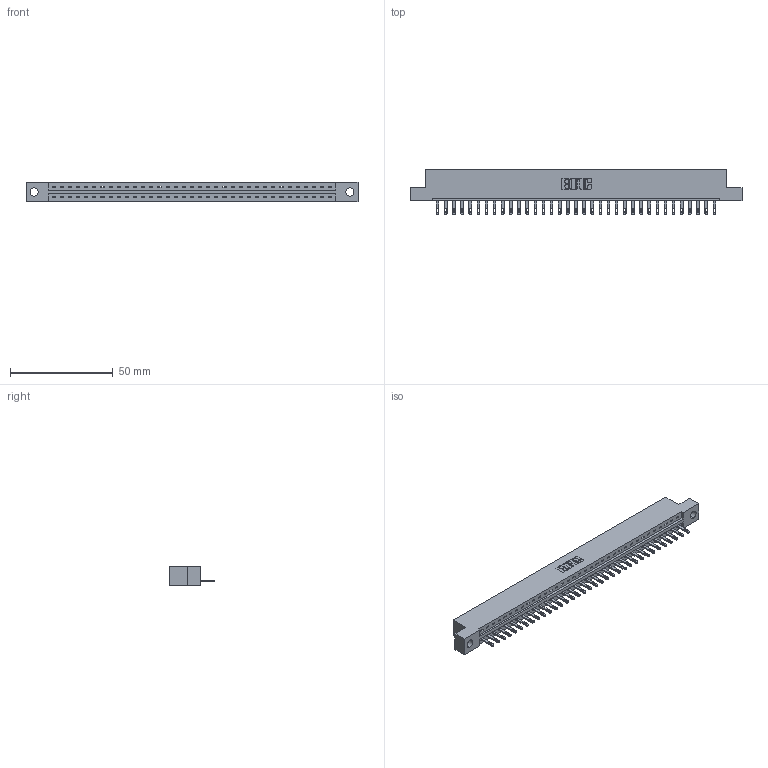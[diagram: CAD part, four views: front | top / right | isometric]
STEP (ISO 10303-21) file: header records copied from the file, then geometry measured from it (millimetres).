
FILE_DESCRIPTION (( 'STEP AP203' ), '1' );
FILE_NAME ('337-035-500-104.STEP', '2019-10-01T12:21:12', ( '' ), ( '' ), 'SwSTEP 2.0', 'SolidWorks 2016', '' );
FILE_SCHEMA (( 'CONFIG_CONTROL_DESIGN' ));
Length unit declared in the file: inch
Products named in the file (3): 337 Part_Flush Mounting Lugs - 0.156 Dia-TH; 337-035-500-104; 345-292-001_345-293-100
Assembly tree (36 placements, depth 2):
  337-035-500-104
    337 Part_Flush Mounting Lugs - 0.156 Dia-TH
    345-292-001_345-293-100  x35
Bounding box: 161.7 x 21.85 x 9.4 mm (x, y, z)
Volume: 16651.8 mm3; surface area: 17045.4 mm2
Topology: 36 solids, 36 shells, 2144 faces, 6611 edges, 4406 vertices
Faces by surface type: plane 1470, cylinder 674
Entity records: 26855 total; most frequent: CARTESIAN_POINT 4683, ORIENTED_EDGE 4654, DIRECTION 3957, EDGE_CURVE 2327, LINE 2195, VECTOR 2195, VERTEX_POINT 1550, AXIS2_PLACEMENT_3D 881
